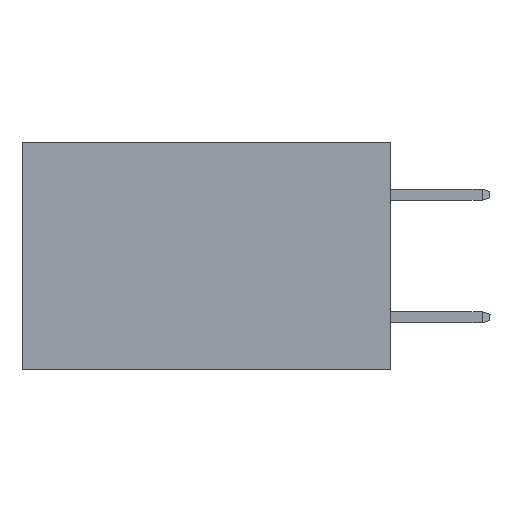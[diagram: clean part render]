
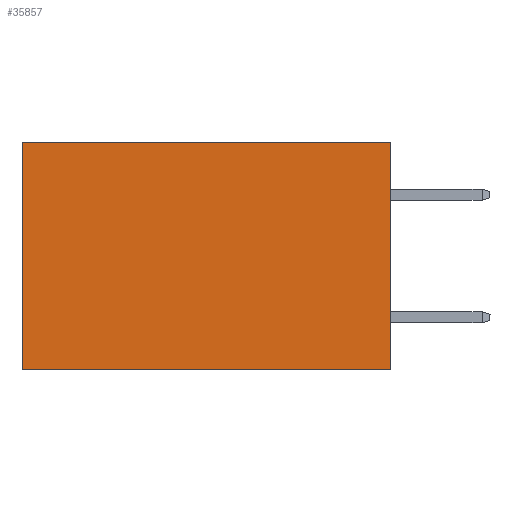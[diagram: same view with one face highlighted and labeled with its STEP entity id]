
A CAD part, left-side view. The second image highlights one B-rep face of the part: STEP entity #35857.
In plain terms, the highlighted planar face has unit normal (-1, 0, 0).
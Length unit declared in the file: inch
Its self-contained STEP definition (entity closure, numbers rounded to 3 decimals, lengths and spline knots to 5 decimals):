
#1545 = VECTOR ( 'NONE', #36131, 39.37008 ) ;
#1683 = CARTESIAN_POINT ( 'NONE',  ( 0.2875, 0.6, 0. ) ) ;
#2243 = CARTESIAN_POINT ( 'NONE',  ( 0.2875, 0., 0. ) ) ;
#3361 = LINE ( 'NONE', #2243, #20755 ) ;
#3959 = VECTOR ( 'NONE', #28184, 39.37008 ) ;
#4290 = VERTEX_POINT ( 'NONE', #24631 ) ;
#7608 = DIRECTION ( 'NONE',  ( 0., 0., -1. ) ) ;
#8881 = CARTESIAN_POINT ( 'NONE',  ( 0.2875, 0., 0. ) ) ;
#9859 = LINE ( 'NONE', #8881, #13741 ) ;
#10703 = ORIENTED_EDGE ( 'NONE', *, *, #24042, .F. ) ;
#11992 = DIRECTION ( 'NONE',  ( 0., 1., 0. ) ) ;
#12421 = EDGE_CURVE ( 'NONE', #4290, #30922, #9859, .T. ) ;
#13741 = VECTOR ( 'NONE', #11992, 39.37008 ) ;
#13963 = PLANE ( 'NONE',  #16484 ) ;
#15065 = ORIENTED_EDGE ( 'NONE', *, *, #39859, .T. ) ;
#15795 = VERTEX_POINT ( 'NONE', #39580 ) ;
#16311 = EDGE_LOOP ( 'NONE', ( #15065, #10703, #18075, #20239 ) ) ;
#16484 = AXIS2_PLACEMENT_3D ( 'NONE', #16939, #19919, #7608 ) ;
#16939 = CARTESIAN_POINT ( 'NONE',  ( 0.2875, 0., 0. ) ) ;
#17558 = CARTESIAN_POINT ( 'NONE',  ( 0.2875, 0.6, 0. ) ) ;
#18075 = ORIENTED_EDGE ( 'NONE', *, *, #20372, .F. ) ;
#18655 = VERTEX_POINT ( 'NONE', #27095 ) ;
#19904 = LINE ( 'NONE', #17558, #1545 ) ;
#19919 = DIRECTION ( 'NONE',  ( 1., 0., 0. ) ) ;
#20239 = ORIENTED_EDGE ( 'NONE', *, *, #12421, .T. ) ;
#20372 = EDGE_CURVE ( 'NONE', #4290, #18655, #3361, .T. ) ;
#20755 = VECTOR ( 'NONE', #38640, 39.37008 ) ;
#21333 = LINE ( 'NONE', #25083, #3959 ) ;
#22596 = FACE_OUTER_BOUND ( 'NONE', #16311, .T. ) ;
#24042 = EDGE_CURVE ( 'NONE', #18655, #15795, #21333, .T. ) ;
#24631 = CARTESIAN_POINT ( 'NONE',  ( 0.2875, 0., 0. ) ) ;
#25083 = CARTESIAN_POINT ( 'NONE',  ( 0.2875, 0., -0.37 ) ) ;
#27095 = CARTESIAN_POINT ( 'NONE',  ( 0.2875, 0., -0.37 ) ) ;
#28184 = DIRECTION ( 'NONE',  ( 0., 1., 0. ) ) ;
#30922 = VERTEX_POINT ( 'NONE', #1683 ) ;
#35857 = ADVANCED_FACE ( 'NONE', ( #22596 ), #13963, .F. ) ;
#36131 = DIRECTION ( 'NONE',  ( 0., 0., -1. ) ) ;
#38640 = DIRECTION ( 'NONE',  ( 0., 0., -1. ) ) ;
#39580 = CARTESIAN_POINT ( 'NONE',  ( 0.2875, 0.6, -0.37 ) ) ;
#39859 = EDGE_CURVE ( 'NONE', #30922, #15795, #19904, .T. ) ;
